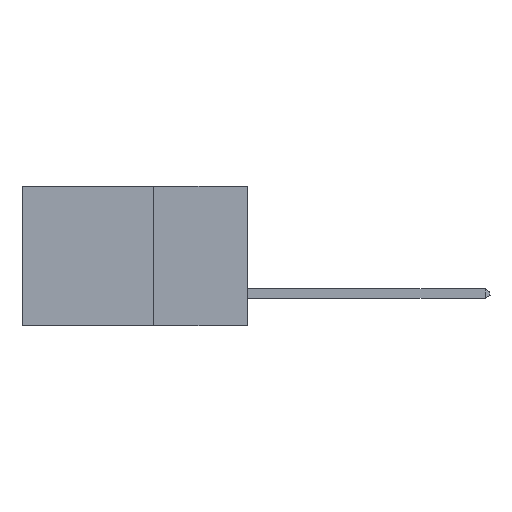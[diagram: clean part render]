
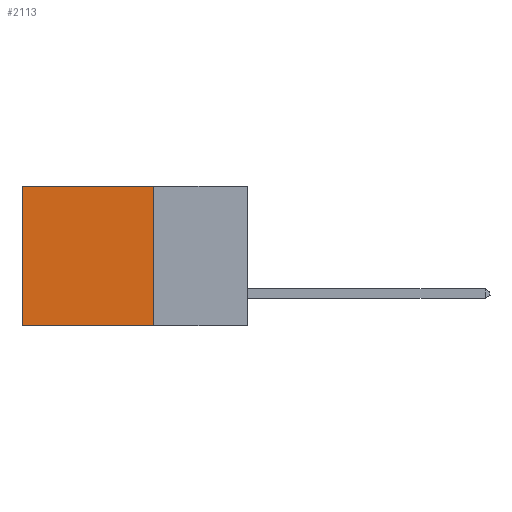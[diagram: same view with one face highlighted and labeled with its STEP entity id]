
A CAD part, left-side view. The second image highlights one B-rep face of the part: STEP entity #2113.
In plain terms, the highlighted planar face has unit normal (-1, 0, 0).
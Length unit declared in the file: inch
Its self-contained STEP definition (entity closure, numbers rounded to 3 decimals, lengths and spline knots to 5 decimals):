
#100 = EDGE_LOOP ( 'NONE', ( #4428, #13923, #15003, #6654 ) ) ;
#128 = PLANE ( 'NONE',  #13174 ) ;
#232 = DIRECTION ( 'NONE',  ( 0., 0., -1. ) ) ;
#457 = CARTESIAN_POINT ( 'NONE',  ( 0.298, 0.25, -0.37 ) ) ;
#2113 = ADVANCED_FACE ( 'NONE', ( #5061 ), #128, .F. ) ;
#2828 = DIRECTION ( 'NONE',  ( 0., 1., 0. ) ) ;
#3191 = EDGE_CURVE ( 'NONE', #9011, #6029, #12110, .T. ) ;
#3197 = DIRECTION ( 'NONE',  ( 0., 0., -1. ) ) ;
#3526 = CARTESIAN_POINT ( 'NONE',  ( 0.298, 0.6, 0. ) ) ;
#4047 = DIRECTION ( 'NONE',  ( 0., 1., 0. ) ) ;
#4069 = VERTEX_POINT ( 'NONE', #14369 ) ;
#4428 = ORIENTED_EDGE ( 'NONE', *, *, #3191, .T. ) ;
#5061 = FACE_OUTER_BOUND ( 'NONE', #100, .T. ) ;
#5522 = VECTOR ( 'NONE', #4047, 39.37008 ) ;
#5695 = CARTESIAN_POINT ( 'NONE',  ( 0.298, 0.25, 0. ) ) ;
#5909 = VECTOR ( 'NONE', #2828, 39.37008 ) ;
#5911 = LINE ( 'NONE', #13683, #5522 ) ;
#6029 = VERTEX_POINT ( 'NONE', #9303 ) ;
#6654 = ORIENTED_EDGE ( 'NONE', *, *, #10481, .T. ) ;
#7274 = VECTOR ( 'NONE', #10910, 39.37008 ) ;
#7545 = CARTESIAN_POINT ( 'NONE',  ( 0.298, 0.25, 0. ) ) ;
#9011 = VERTEX_POINT ( 'NONE', #9118 ) ;
#9118 = CARTESIAN_POINT ( 'NONE',  ( 0.298, 0.6, 0. ) ) ;
#9303 = CARTESIAN_POINT ( 'NONE',  ( 0.298, 0.6, -0.37 ) ) ;
#9859 = EDGE_CURVE ( 'NONE', #11505, #6029, #12075, .T. ) ;
#10481 = EDGE_CURVE ( 'NONE', #4069, #9011, #5911, .T. ) ;
#10682 = LINE ( 'NONE', #5695, #11459 ) ;
#10910 = DIRECTION ( 'NONE',  ( 0., 0., -1. ) ) ;
#11003 = EDGE_CURVE ( 'NONE', #4069, #11505, #10682, .T. ) ;
#11459 = VECTOR ( 'NONE', #3197, 39.37008 ) ;
#11505 = VERTEX_POINT ( 'NONE', #457 ) ;
#12075 = LINE ( 'NONE', #15191, #5909 ) ;
#12110 = LINE ( 'NONE', #3526, #7274 ) ;
#12497 = DIRECTION ( 'NONE',  ( 1., 0., 0. ) ) ;
#13174 = AXIS2_PLACEMENT_3D ( 'NONE', #7545, #12497, #232 ) ;
#13683 = CARTESIAN_POINT ( 'NONE',  ( 0.298, 0.25, 0. ) ) ;
#13923 = ORIENTED_EDGE ( 'NONE', *, *, #9859, .F. ) ;
#14369 = CARTESIAN_POINT ( 'NONE',  ( 0.298, 0.25, 0. ) ) ;
#15003 = ORIENTED_EDGE ( 'NONE', *, *, #11003, .F. ) ;
#15191 = CARTESIAN_POINT ( 'NONE',  ( 0.298, 0.25, -0.37 ) ) ;
